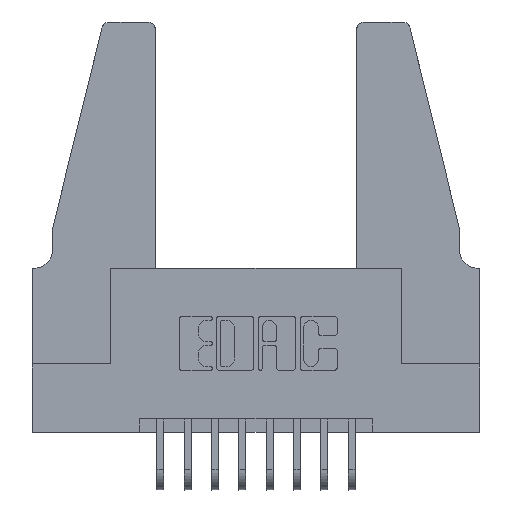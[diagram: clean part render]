
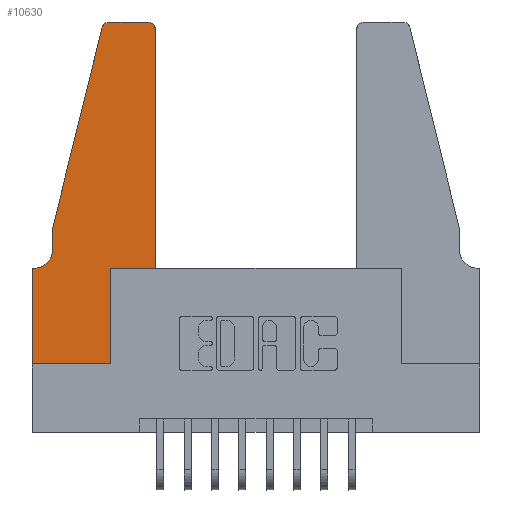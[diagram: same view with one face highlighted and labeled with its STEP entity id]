
A CAD part, top view. The second image highlights one B-rep face of the part: STEP entity #10630.
In plain terms, the highlighted planar face has unit normal (0, 0, 1).
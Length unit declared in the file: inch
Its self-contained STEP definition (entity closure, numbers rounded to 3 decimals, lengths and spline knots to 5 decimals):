
#40 = DIRECTION ( 'NONE',  ( -1., 0., 0. ) ) ;
#172 = VERTEX_POINT ( 'NONE', #8139 ) ;
#444 = VECTOR ( 'NONE', #9069, 39.37008 ) ;
#461 = PLANE ( 'NONE',  #7256 ) ;
#538 = VECTOR ( 'NONE', #13378, 39.37008 ) ;
#541 = VECTOR ( 'NONE', #40, 39.37008 ) ;
#1115 = DIRECTION ( 'NONE',  ( 1., 0., 0. ) ) ;
#1154 = CARTESIAN_POINT ( 'NONE',  ( 0.4505, 0.35, 0.37 ) ) ;
#1245 = EDGE_CURVE ( 'NONE', #172, #13972, #5734, .T. ) ;
#1346 = CARTESIAN_POINT ( 'NONE',  ( 0.2865, 0., 0.37 ) ) ;
#1432 = VERTEX_POINT ( 'NONE', #14118 ) ;
#1524 = DIRECTION ( 'NONE',  ( 0., -1., 0. ) ) ;
#1775 = DIRECTION ( 'NONE',  ( -1., 0., 0. ) ) ;
#1890 = CARTESIAN_POINT ( 'NONE',  ( 0.0755, 0.42, 0.37 ) ) ;
#1978 = CARTESIAN_POINT ( 'NONE',  ( 0., 0., 0.37 ) ) ;
#2072 = CARTESIAN_POINT ( 'NONE',  ( 0.4505, 0.35, 0.37 ) ) ;
#2085 = LINE ( 'NONE', #9644, #10754 ) ;
#2122 = VERTEX_POINT ( 'NONE', #14585 ) ;
#2155 = EDGE_CURVE ( 'NONE', #12896, #6020, #3056, .T. ) ;
#2361 = VECTOR ( 'NONE', #1524, 39.37008 ) ;
#2595 = FACE_OUTER_BOUND ( 'NONE', #8117, .T. ) ;
#2795 = VERTEX_POINT ( 'NONE', #8816 ) ;
#2875 = VERTEX_POINT ( 'NONE', #4612 ) ;
#3056 = LINE ( 'NONE', #11084, #538 ) ;
#3085 = CIRCLE ( 'NONE', #8453, 0.03 ) ;
#3096 = VECTOR ( 'NONE', #11771, 39.37008 ) ;
#3158 = CARTESIAN_POINT ( 'NONE',  ( 0., 0.35, 0.37 ) ) ;
#3167 = LINE ( 'NONE', #7271, #6701 ) ;
#3217 = EDGE_CURVE ( 'NONE', #2795, #1432, #8875, .T. ) ;
#3489 = LINE ( 'NONE', #12778, #11438 ) ;
#3526 = DIRECTION ( 'NONE',  ( 0., 0., -1. ) ) ;
#3548 = EDGE_CURVE ( 'NONE', #6398, #5565, #12593, .T. ) ;
#3586 = ORIENTED_EDGE ( 'NONE', *, *, #12541, .T. ) ;
#3689 = ORIENTED_EDGE ( 'NONE', *, *, #8195, .T. ) ;
#3915 = AXIS2_PLACEMENT_3D ( 'NONE', #13828, #3526, #12578 ) ;
#3966 = CARTESIAN_POINT ( 'NONE',  ( 0.0755, 0.5, 0.37 ) ) ;
#4206 = VERTEX_POINT ( 'NONE', #3158 ) ;
#4415 = ORIENTED_EDGE ( 'NONE', *, *, #5962, .T. ) ;
#4612 = CARTESIAN_POINT ( 'NONE',  ( 0.2865, 0.35, 0.37 ) ) ;
#4815 = DIRECTION ( 'NONE',  ( 1., 0., 0. ) ) ;
#5341 = ORIENTED_EDGE ( 'NONE', *, *, #5406, .T. ) ;
#5406 = EDGE_CURVE ( 'NONE', #4206, #12896, #2085, .T. ) ;
#5565 = VERTEX_POINT ( 'NONE', #7013 ) ;
#5664 = CARTESIAN_POINT ( 'NONE',  ( 0.2865, 0.35, 0.37 ) ) ;
#5734 = LINE ( 'NONE', #3966, #2361 ) ;
#5819 = CARTESIAN_POINT ( 'NONE',  ( 0.2605, 1.25, 0.37 ) ) ;
#5962 = EDGE_CURVE ( 'NONE', #5565, #2795, #14672, .T. ) ;
#6020 = VERTEX_POINT ( 'NONE', #1346 ) ;
#6102 = ORIENTED_EDGE ( 'NONE', *, *, #11262, .T. ) ;
#6398 = VERTEX_POINT ( 'NONE', #12171 ) ;
#6426 = ORIENTED_EDGE ( 'NONE', *, *, #1245, .T. ) ;
#6489 = LINE ( 'NONE', #1154, #444 ) ;
#6701 = VECTOR ( 'NONE', #1775, 39.37008 ) ;
#6809 = LINE ( 'NONE', #5664, #3096 ) ;
#7013 = CARTESIAN_POINT ( 'NONE',  ( 0.4505, 1.22, 0.37 ) ) ;
#7027 = EDGE_CURVE ( 'NONE', #9792, #172, #3489, .T. ) ;
#7256 = AXIS2_PLACEMENT_3D ( 'NONE', #13918, #10218, #7360 ) ;
#7271 = CARTESIAN_POINT ( 'NONE',  ( 0.0755, 0.35, 0.37 ) ) ;
#7360 = DIRECTION ( 'NONE',  ( 1., 0., 0. ) ) ;
#7384 = DIRECTION ( 'NONE',  ( 0., -1., 0. ) ) ;
#8113 = ORIENTED_EDGE ( 'NONE', *, *, #2155, .T. ) ;
#8117 = EDGE_LOOP ( 'NONE', ( #12403, #13659, #10865, #6426, #3689, #14690, #5341, #8113, #3586, #6102, #14552, #4415 ) ) ;
#8139 = CARTESIAN_POINT ( 'NONE',  ( 0.0755, 0.5, 0.37 ) ) ;
#8161 = DIRECTION ( 'NONE',  ( 0., 0., 1. ) ) ;
#8195 = EDGE_CURVE ( 'NONE', #13972, #2122, #13007, .T. ) ;
#8453 = AXIS2_PLACEMENT_3D ( 'NONE', #10226, #9178, #1115 ) ;
#8679 = EDGE_CURVE ( 'NONE', #1432, #9792, #3085, .T. ) ;
#8816 = CARTESIAN_POINT ( 'NONE',  ( 0.4205, 1.25, 0.37 ) ) ;
#8875 = LINE ( 'NONE', #5819, #541 ) ;
#9069 = DIRECTION ( 'NONE',  ( 1., 0., 0. ) ) ;
#9178 = DIRECTION ( 'NONE',  ( 0., 0., 1. ) ) ;
#9504 = DIRECTION ( 'NONE',  ( -0.239, -0.971, 0. ) ) ;
#9644 = CARTESIAN_POINT ( 'NONE',  ( 0., 0., 0.37 ) ) ;
#9792 = VERTEX_POINT ( 'NONE', #12322 ) ;
#9973 = DIRECTION ( 'NONE',  ( 0., 1., 0. ) ) ;
#10218 = DIRECTION ( 'NONE',  ( 0., 0., 1. ) ) ;
#10226 = CARTESIAN_POINT ( 'NONE',  ( 0.284, 1.22, 0.37 ) ) ;
#10365 = EDGE_CURVE ( 'NONE', #2122, #4206, #3167, .T. ) ;
#10630 = ADVANCED_FACE ( 'NONE', ( #2595 ), #461, .T. ) ;
#10754 = VECTOR ( 'NONE', #7384, 39.37008 ) ;
#10865 = ORIENTED_EDGE ( 'NONE', *, *, #7027, .T. ) ;
#11084 = CARTESIAN_POINT ( 'NONE',  ( 0., 0., 0.37 ) ) ;
#11262 = EDGE_CURVE ( 'NONE', #2875, #6398, #6489, .T. ) ;
#11438 = VECTOR ( 'NONE', #9504, 39.37008 ) ;
#11500 = CARTESIAN_POINT ( 'NONE',  ( 0.4205, 1.22, 0.37 ) ) ;
#11771 = DIRECTION ( 'NONE',  ( 0., 1., 0. ) ) ;
#12171 = CARTESIAN_POINT ( 'NONE',  ( 0.4505, 0.35, 0.37 ) ) ;
#12322 = CARTESIAN_POINT ( 'NONE',  ( 0.25487, 1.22718, 0.37 ) ) ;
#12403 = ORIENTED_EDGE ( 'NONE', *, *, #3217, .T. ) ;
#12541 = EDGE_CURVE ( 'NONE', #6020, #2875, #6809, .T. ) ;
#12578 = DIRECTION ( 'NONE',  ( -1., 0., 0. ) ) ;
#12593 = LINE ( 'NONE', #2072, #13312 ) ;
#12778 = CARTESIAN_POINT ( 'NONE',  ( 0.0755, 0.5, 0.37 ) ) ;
#12896 = VERTEX_POINT ( 'NONE', #1978 ) ;
#13007 = CIRCLE ( 'NONE', #3915, 0.07 ) ;
#13312 = VECTOR ( 'NONE', #9973, 39.37008 ) ;
#13378 = DIRECTION ( 'NONE',  ( 1., 0., 0. ) ) ;
#13659 = ORIENTED_EDGE ( 'NONE', *, *, #8679, .T. ) ;
#13828 = CARTESIAN_POINT ( 'NONE',  ( 0.0055, 0.42, 0.37 ) ) ;
#13918 = CARTESIAN_POINT ( 'NONE',  ( 0., 0.35, 0.37 ) ) ;
#13972 = VERTEX_POINT ( 'NONE', #1890 ) ;
#14069 = AXIS2_PLACEMENT_3D ( 'NONE', #11500, #8161, #4815 ) ;
#14118 = CARTESIAN_POINT ( 'NONE',  ( 0.284, 1.25, 0.37 ) ) ;
#14552 = ORIENTED_EDGE ( 'NONE', *, *, #3548, .T. ) ;
#14585 = CARTESIAN_POINT ( 'NONE',  ( 0.0055, 0.35, 0.37 ) ) ;
#14672 = CIRCLE ( 'NONE', #14069, 0.03 ) ;
#14690 = ORIENTED_EDGE ( 'NONE', *, *, #10365, .T. ) ;
